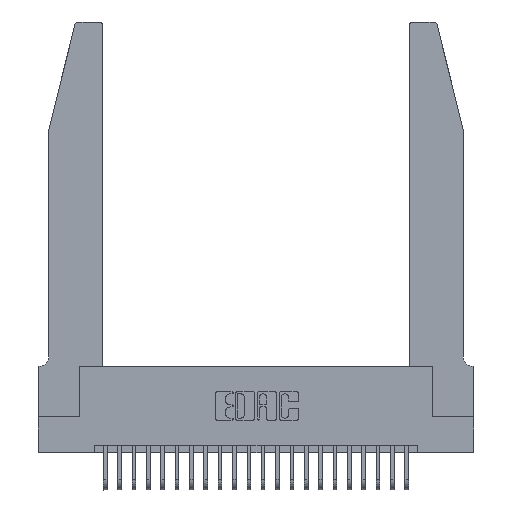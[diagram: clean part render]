
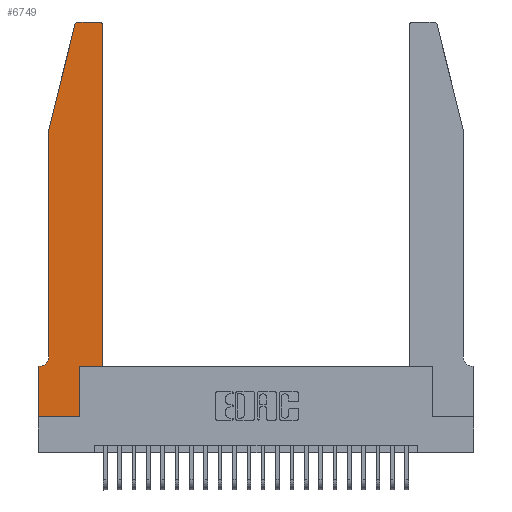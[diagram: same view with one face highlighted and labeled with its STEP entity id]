
A CAD part, top view. The second image highlights one B-rep face of the part: STEP entity #6749.
In plain terms, the highlighted planar face has unit normal (0, 0, 1).
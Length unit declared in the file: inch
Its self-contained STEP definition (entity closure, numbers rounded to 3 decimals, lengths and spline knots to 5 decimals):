
#25 = LINE ( 'NONE', #1238, #13751 ) ;
#216 = DIRECTION ( 'NONE',  ( 0., -1., 0. ) ) ;
#251 = DIRECTION ( 'NONE',  ( 1., 0., 0. ) ) ;
#521 = VERTEX_POINT ( 'NONE', #16367 ) ;
#696 = DIRECTION ( 'NONE',  ( 1., 0., 0. ) ) ;
#746 = EDGE_CURVE ( 'NONE', #521, #2874, #19199, .T. ) ;
#802 = VERTEX_POINT ( 'NONE', #8752 ) ;
#1103 = EDGE_CURVE ( 'NONE', #2874, #18577, #21500, .T. ) ;
#1238 = CARTESIAN_POINT ( 'NONE',  ( 0.0755, 2., 0.37 ) ) ;
#1360 = CARTESIAN_POINT ( 'NONE',  ( 0., 0., 0.37 ) ) ;
#1420 = CARTESIAN_POINT ( 'NONE',  ( 0.0755, 0.42, 0.37 ) ) ;
#1534 = CARTESIAN_POINT ( 'NONE',  ( 0.0755, 0.35, 0.37 ) ) ;
#1541 = DIRECTION ( 'NONE',  ( 0., 1., 0. ) ) ;
#1545 = DIRECTION ( 'NONE',  ( 0., -1., 0. ) ) ;
#2044 = EDGE_LOOP ( 'NONE', ( #7653, #21781, #5323, #18667, #11988, #8187, #9975, #5597, #15507, #2981, #18422, #19564 ) ) ;
#2531 = EDGE_CURVE ( 'NONE', #12495, #20487, #7160, .T. ) ;
#2874 = VERTEX_POINT ( 'NONE', #12440 ) ;
#2981 = ORIENTED_EDGE ( 'NONE', *, *, #10250, .T. ) ;
#3049 = EDGE_CURVE ( 'NONE', #16932, #521, #20810, .T. ) ;
#3444 = VECTOR ( 'NONE', #1541, 39.37008 ) ;
#4232 = LINE ( 'NONE', #10840, #23415 ) ;
#4266 = CARTESIAN_POINT ( 'NONE',  ( 0.2865, 0.35, 0.37 ) ) ;
#5048 = CARTESIAN_POINT ( 'NONE',  ( 0., 0.35, 0.37 ) ) ;
#5093 = AXIS2_PLACEMENT_3D ( 'NONE', #11316, #11211, #14399 ) ;
#5323 = ORIENTED_EDGE ( 'NONE', *, *, #11111, .T. ) ;
#5597 = ORIENTED_EDGE ( 'NONE', *, *, #17655, .T. ) ;
#5830 = CARTESIAN_POINT ( 'NONE',  ( 0.4505, 0.35, 0.37 ) ) ;
#5853 = EDGE_CURVE ( 'NONE', #802, #19659, #19496, .T. ) ;
#6749 = ADVANCED_FACE ( 'NONE', ( #19445 ), #16212, .T. ) ;
#6828 = EDGE_CURVE ( 'NONE', #14145, #16932, #23205, .T. ) ;
#6915 = DIRECTION ( 'NONE',  ( 0., 0., 1. ) ) ;
#7160 = CIRCLE ( 'NONE', #5093, 0.07 ) ;
#7653 = ORIENTED_EDGE ( 'NONE', *, *, #746, .T. ) ;
#7835 = DIRECTION ( 'NONE',  ( -1., 0., 0. ) ) ;
#8187 = ORIENTED_EDGE ( 'NONE', *, *, #11899, .T. ) ;
#8496 = VECTOR ( 'NONE', #696, 39.37008 ) ;
#8752 = CARTESIAN_POINT ( 'NONE',  ( 0.2865, 0., 0.37 ) ) ;
#8905 = VERTEX_POINT ( 'NONE', #20775 ) ;
#9542 = CARTESIAN_POINT ( 'NONE',  ( 0.0755, 2., 0.37 ) ) ;
#9660 = VERTEX_POINT ( 'NONE', #13856 ) ;
#9975 = ORIENTED_EDGE ( 'NONE', *, *, #19418, .T. ) ;
#10250 = EDGE_CURVE ( 'NONE', #19659, #14145, #18408, .T. ) ;
#10536 = CARTESIAN_POINT ( 'NONE',  ( 0.2605, 2.75, 0.37 ) ) ;
#10840 = CARTESIAN_POINT ( 'NONE',  ( 0., 0., 0.37 ) ) ;
#11111 = EDGE_CURVE ( 'NONE', #18577, #9660, #25, .T. ) ;
#11211 = DIRECTION ( 'NONE',  ( 0., 0., -1. ) ) ;
#11316 = CARTESIAN_POINT ( 'NONE',  ( 0.0055, 0.42, 0.37 ) ) ;
#11457 = DIRECTION ( 'NONE',  ( 0., 0., 1. ) ) ;
#11880 = CARTESIAN_POINT ( 'NONE',  ( 0.4505, 0.35, 0.37 ) ) ;
#11899 = EDGE_CURVE ( 'NONE', #20487, #13193, #12855, .T. ) ;
#11988 = ORIENTED_EDGE ( 'NONE', *, *, #2531, .T. ) ;
#12264 = VECTOR ( 'NONE', #21946, 39.37008 ) ;
#12422 = CARTESIAN_POINT ( 'NONE',  ( 0.4505, 2.72, 0.37 ) ) ;
#12440 = CARTESIAN_POINT ( 'NONE',  ( 0.284, 2.75, 0.37 ) ) ;
#12495 = VERTEX_POINT ( 'NONE', #1420 ) ;
#12736 = CARTESIAN_POINT ( 'NONE',  ( 0.284, 2.72, 0.37 ) ) ;
#12855 = LINE ( 'NONE', #1534, #12264 ) ;
#13193 = VERTEX_POINT ( 'NONE', #20343 ) ;
#13312 = EDGE_CURVE ( 'NONE', #9660, #12495, #22636, .T. ) ;
#13662 = VECTOR ( 'NONE', #19996, 39.37008 ) ;
#13741 = DIRECTION ( 'NONE',  ( 1., 0., 0. ) ) ;
#13751 = VECTOR ( 'NONE', #23581, 39.37008 ) ;
#13856 = CARTESIAN_POINT ( 'NONE',  ( 0.0755, 2., 0.37 ) ) ;
#14145 = VERTEX_POINT ( 'NONE', #5830 ) ;
#14399 = DIRECTION ( 'NONE',  ( -1., 0., 0. ) ) ;
#14584 = VECTOR ( 'NONE', #19149, 39.37008 ) ;
#14921 = AXIS2_PLACEMENT_3D ( 'NONE', #12736, #18887, #13741 ) ;
#15339 = CARTESIAN_POINT ( 'NONE',  ( 0.25487, 2.72718, 0.37 ) ) ;
#15507 = ORIENTED_EDGE ( 'NONE', *, *, #5853, .T. ) ;
#16212 = PLANE ( 'NONE',  #18569 ) ;
#16367 = CARTESIAN_POINT ( 'NONE',  ( 0.4205, 2.75, 0.37 ) ) ;
#16932 = VERTEX_POINT ( 'NONE', #12422 ) ;
#17655 = EDGE_CURVE ( 'NONE', #8905, #802, #18596, .T. ) ;
#18408 = LINE ( 'NONE', #11880, #8496 ) ;
#18422 = ORIENTED_EDGE ( 'NONE', *, *, #6828, .T. ) ;
#18569 = AXIS2_PLACEMENT_3D ( 'NONE', #5048, #6915, #19930 ) ;
#18577 = VERTEX_POINT ( 'NONE', #15339 ) ;
#18596 = LINE ( 'NONE', #1360, #13662 ) ;
#18626 = VECTOR ( 'NONE', #7835, 39.37008 ) ;
#18667 = ORIENTED_EDGE ( 'NONE', *, *, #13312, .T. ) ;
#18887 = DIRECTION ( 'NONE',  ( 0., 0., 1. ) ) ;
#19149 = DIRECTION ( 'NONE',  ( 0., 1., 0. ) ) ;
#19199 = LINE ( 'NONE', #10536, #18626 ) ;
#19418 = EDGE_CURVE ( 'NONE', #13193, #8905, #4232, .T. ) ;
#19445 = FACE_OUTER_BOUND ( 'NONE', #2044, .T. ) ;
#19496 = LINE ( 'NONE', #4266, #14584 ) ;
#19564 = ORIENTED_EDGE ( 'NONE', *, *, #3049, .T. ) ;
#19659 = VERTEX_POINT ( 'NONE', #20814 ) ;
#19930 = DIRECTION ( 'NONE',  ( 1., 0., 0. ) ) ;
#19996 = DIRECTION ( 'NONE',  ( 1., 0., 0. ) ) ;
#20343 = CARTESIAN_POINT ( 'NONE',  ( 0., 0.35, 0.37 ) ) ;
#20487 = VERTEX_POINT ( 'NONE', #23593 ) ;
#20775 = CARTESIAN_POINT ( 'NONE',  ( 0., 0., 0.37 ) ) ;
#20810 = CIRCLE ( 'NONE', #23293, 0.03 ) ;
#20814 = CARTESIAN_POINT ( 'NONE',  ( 0.2865, 0.35, 0.37 ) ) ;
#20892 = VECTOR ( 'NONE', #216, 39.37008 ) ;
#21500 = CIRCLE ( 'NONE', #14921, 0.03 ) ;
#21781 = ORIENTED_EDGE ( 'NONE', *, *, #1103, .T. ) ;
#21946 = DIRECTION ( 'NONE',  ( -1., 0., 0. ) ) ;
#21956 = CARTESIAN_POINT ( 'NONE',  ( 0.4505, 0.35, 0.37 ) ) ;
#22564 = CARTESIAN_POINT ( 'NONE',  ( 0.4205, 2.72, 0.37 ) ) ;
#22636 = LINE ( 'NONE', #9542, #20892 ) ;
#23205 = LINE ( 'NONE', #21956, #3444 ) ;
#23293 = AXIS2_PLACEMENT_3D ( 'NONE', #22564, #11457, #251 ) ;
#23415 = VECTOR ( 'NONE', #1545, 39.37008 ) ;
#23581 = DIRECTION ( 'NONE',  ( -0.239, -0.971, 0. ) ) ;
#23593 = CARTESIAN_POINT ( 'NONE',  ( 0.0055, 0.35, 0.37 ) ) ;
